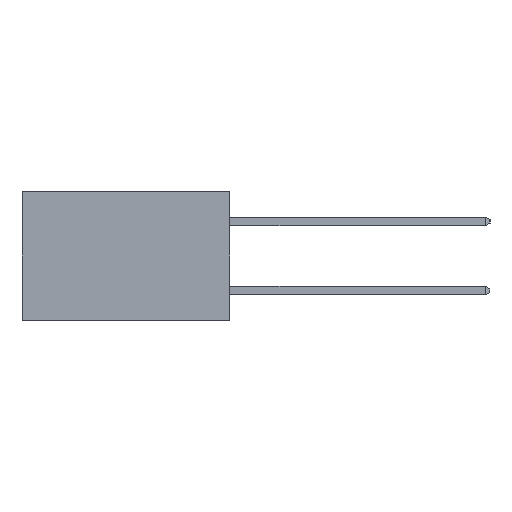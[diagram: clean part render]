
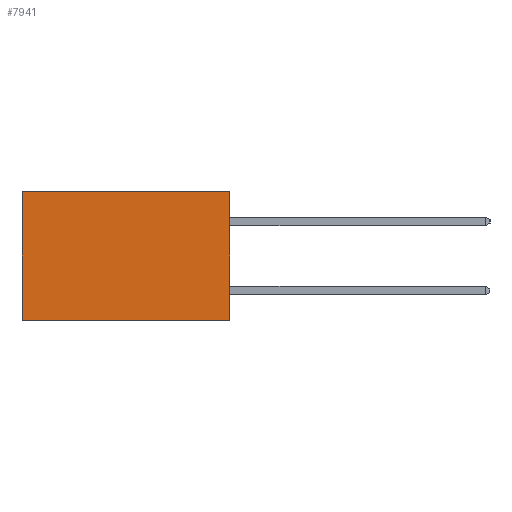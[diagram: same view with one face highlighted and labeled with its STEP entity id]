
A CAD part, left-side view. The second image highlights one B-rep face of the part: STEP entity #7941.
In plain terms, the highlighted planar face has unit normal (-1, 0, 0).
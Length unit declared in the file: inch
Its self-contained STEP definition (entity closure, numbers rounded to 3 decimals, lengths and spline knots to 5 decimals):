
#106 = EDGE_CURVE ( 'NONE', #5039, #8732, #6796, .T. ) ;
#227 = EDGE_CURVE ( 'NONE', #8732, #8960, #2012, .T. ) ;
#1550 = CARTESIAN_POINT ( 'NONE',  ( 0.298, 0.6, -0.37 ) ) ;
#1890 = DIRECTION ( 'NONE',  ( 0., 0., -1. ) ) ;
#1944 = CARTESIAN_POINT ( 'NONE',  ( 0.298, 0., 0. ) ) ;
#2012 = LINE ( 'NONE', #9191, #5946 ) ;
#2682 = CARTESIAN_POINT ( 'NONE',  ( 0.298, 0.6, 0. ) ) ;
#2725 = LINE ( 'NONE', #2682, #4852 ) ;
#3663 = CARTESIAN_POINT ( 'NONE',  ( 0.298, 0., 0. ) ) ;
#4226 = CARTESIAN_POINT ( 'NONE',  ( 0.298, 0.6, 0. ) ) ;
#4249 = DIRECTION ( 'NONE',  ( 1., 0., 0. ) ) ;
#4276 = DIRECTION ( 'NONE',  ( 0., 0., -1. ) ) ;
#4480 = EDGE_CURVE ( 'NONE', #4512, #8960, #2725, .T. ) ;
#4512 = VERTEX_POINT ( 'NONE', #4226 ) ;
#4852 = VECTOR ( 'NONE', #4276, 39.37008 ) ;
#5039 = VERTEX_POINT ( 'NONE', #3663 ) ;
#5888 = ORIENTED_EDGE ( 'NONE', *, *, #4480, .T. ) ;
#5896 = ORIENTED_EDGE ( 'NONE', *, *, #227, .F. ) ;
#5945 = ORIENTED_EDGE ( 'NONE', *, *, #106, .F. ) ;
#5946 = VECTOR ( 'NONE', #9664, 39.37008 ) ;
#5957 = ORIENTED_EDGE ( 'NONE', *, *, #7087, .T. ) ;
#6647 = CARTESIAN_POINT ( 'NONE',  ( 0.298, 0., 0. ) ) ;
#6796 = LINE ( 'NONE', #1944, #8455 ) ;
#7053 = VECTOR ( 'NONE', #7492, 39.37008 ) ;
#7074 = EDGE_LOOP ( 'NONE', ( #5888, #5896, #5945, #5957 ) ) ;
#7087 = EDGE_CURVE ( 'NONE', #5039, #4512, #9051, .T. ) ;
#7284 = CARTESIAN_POINT ( 'NONE',  ( 0.298, 0., 0. ) ) ;
#7492 = DIRECTION ( 'NONE',  ( 0., 1., 0. ) ) ;
#7941 = ADVANCED_FACE ( 'NONE', ( #9988 ), #8165, .F. ) ;
#8165 = PLANE ( 'NONE',  #9225 ) ;
#8455 = VECTOR ( 'NONE', #1890, 39.37008 ) ;
#8732 = VERTEX_POINT ( 'NONE', #9809 ) ;
#8960 = VERTEX_POINT ( 'NONE', #1550 ) ;
#9051 = LINE ( 'NONE', #6647, #7053 ) ;
#9191 = CARTESIAN_POINT ( 'NONE',  ( 0.298, 0., -0.37 ) ) ;
#9225 = AXIS2_PLACEMENT_3D ( 'NONE', #7284, #4249, #9447 ) ;
#9447 = DIRECTION ( 'NONE',  ( 0., 0., -1. ) ) ;
#9664 = DIRECTION ( 'NONE',  ( 0., 1., 0. ) ) ;
#9809 = CARTESIAN_POINT ( 'NONE',  ( 0.298, 0., -0.37 ) ) ;
#9988 = FACE_OUTER_BOUND ( 'NONE', #7074, .T. ) ;
